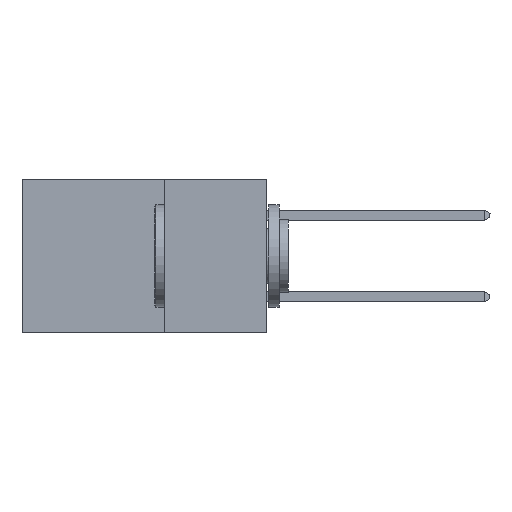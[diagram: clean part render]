
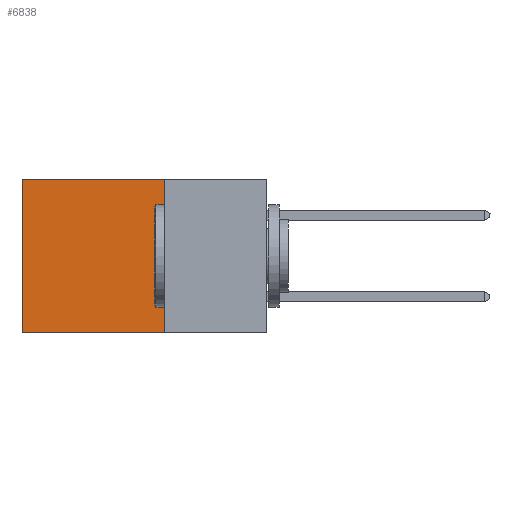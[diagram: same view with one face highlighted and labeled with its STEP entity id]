
A CAD part, left-side view. The second image highlights one B-rep face of the part: STEP entity #6838.
In plain terms, the highlighted planar face has unit normal (-1, 0, 0).
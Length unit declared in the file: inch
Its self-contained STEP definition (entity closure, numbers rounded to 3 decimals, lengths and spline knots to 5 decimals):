
#532 = DIRECTION ( 'NONE',  ( 0., 1., 0. ) ) ;
#1001 = CARTESIAN_POINT ( 'NONE',  ( 0.2875, 0.25, -0.375 ) ) ;
#1004 = VECTOR ( 'NONE', #10026, 39.37008 ) ;
#1219 = CARTESIAN_POINT ( 'NONE',  ( 0.2875, 0.25, 0. ) ) ;
#1403 = VERTEX_POINT ( 'NONE', #1219 ) ;
#1546 = ORIENTED_EDGE ( 'NONE', *, *, #4807, .T. ) ;
#1899 = VERTEX_POINT ( 'NONE', #3668 ) ;
#2214 = VERTEX_POINT ( 'NONE', #1001 ) ;
#2310 = VECTOR ( 'NONE', #10398, 39.37008 ) ;
#2855 = CARTESIAN_POINT ( 'NONE',  ( 0.2875, 0.25, -0.375 ) ) ;
#3026 = DIRECTION ( 'NONE',  ( 1., 0., 0. ) ) ;
#3467 = LINE ( 'NONE', #7883, #7274 ) ;
#3506 = CARTESIAN_POINT ( 'NONE',  ( 0.2875, 0.6, -0.375 ) ) ;
#3596 = VECTOR ( 'NONE', #532, 39.37008 ) ;
#3668 = CARTESIAN_POINT ( 'NONE',  ( 0.2875, 0.6, 0. ) ) ;
#3722 = LINE ( 'NONE', #6912, #2310 ) ;
#3994 = EDGE_LOOP ( 'NONE', ( #8745, #8519, #7923, #1546 ) ) ;
#4035 = AXIS2_PLACEMENT_3D ( 'NONE', #10694, #3026, #7441 ) ;
#4143 = CARTESIAN_POINT ( 'NONE',  ( 0.2875, 0.6, -0.375 ) ) ;
#4807 = EDGE_CURVE ( 'NONE', #1403, #1899, #3467, .T. ) ;
#6275 = FACE_OUTER_BOUND ( 'NONE', #3994, .T. ) ;
#6650 = DIRECTION ( 'NONE',  ( 0., 1., 0. ) ) ;
#6838 = ADVANCED_FACE ( 'NONE', ( #6275 ), #7308, .F. ) ;
#6912 = CARTESIAN_POINT ( 'NONE',  ( 0.2875, 0.25, -0.375 ) ) ;
#7274 = VECTOR ( 'NONE', #6650, 39.37008 ) ;
#7308 = PLANE ( 'NONE',  #4035 ) ;
#7441 = DIRECTION ( 'NONE',  ( 0., 0., -1. ) ) ;
#7701 = LINE ( 'NONE', #3506, #1004 ) ;
#7710 = VERTEX_POINT ( 'NONE', #4143 ) ;
#7883 = CARTESIAN_POINT ( 'NONE',  ( 0.2875, 0.25, 0. ) ) ;
#7923 = ORIENTED_EDGE ( 'NONE', *, *, #10266, .F. ) ;
#8519 = ORIENTED_EDGE ( 'NONE', *, *, #13872, .F. ) ;
#8723 = EDGE_CURVE ( 'NONE', #1899, #7710, #7701, .T. ) ;
#8745 = ORIENTED_EDGE ( 'NONE', *, *, #8723, .T. ) ;
#10026 = DIRECTION ( 'NONE',  ( 0., 0., -1. ) ) ;
#10266 = EDGE_CURVE ( 'NONE', #1403, #2214, #3722, .T. ) ;
#10398 = DIRECTION ( 'NONE',  ( 0., 0., -1. ) ) ;
#10694 = CARTESIAN_POINT ( 'NONE',  ( 0.2875, 0.25, -0.375 ) ) ;
#10742 = LINE ( 'NONE', #2855, #3596 ) ;
#13872 = EDGE_CURVE ( 'NONE', #2214, #7710, #10742, .T. ) ;
